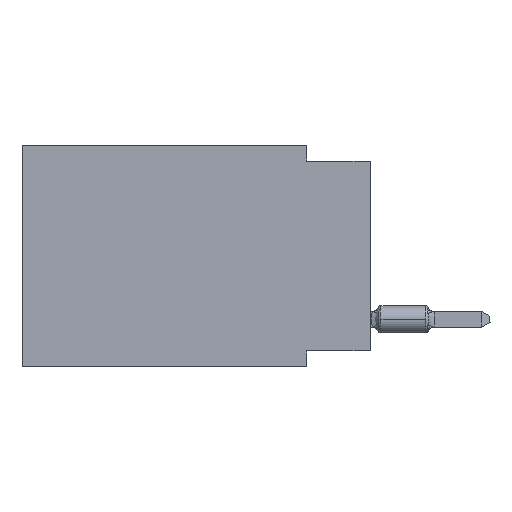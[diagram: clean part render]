
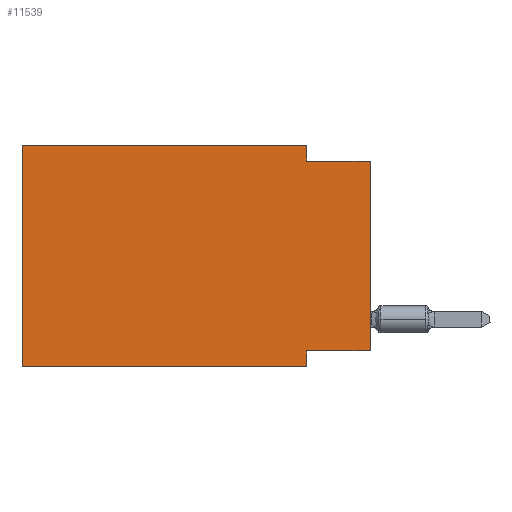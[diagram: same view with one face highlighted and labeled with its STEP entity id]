
A CAD part, left-side view. The second image highlights one B-rep face of the part: STEP entity #11539.
In plain terms, the highlighted planar face has unit normal (-1, 0, 0).
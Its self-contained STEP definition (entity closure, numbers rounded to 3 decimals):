
#651 = DIRECTION ( 'NONE',  ( 0., -1., 0. ) ) ;
#812 = VECTOR ( 'NONE', #651, 1000. ) ;
#1821 = DIRECTION ( 'NONE',  ( 0., -1., 0. ) ) ;
#2051 = LINE ( 'NONE', #42068, #29539 ) ;
#3087 = ORIENTED_EDGE ( 'NONE', *, *, #17412, .F. ) ;
#3097 = AXIS2_PLACEMENT_3D ( 'NONE', #10239, #26311, #42334 ) ;
#3133 = DIRECTION ( 'NONE',  ( 0., 1., 0. ) ) ;
#3184 = DIRECTION ( 'NONE',  ( 0., 0., -1. ) ) ;
#4535 = CARTESIAN_POINT ( 'NONE',  ( 0., 13.97, 0. ) ) ;
#7251 = VECTOR ( 'NONE', #44217, 1000. ) ;
#7357 = LINE ( 'NONE', #51108, #7251 ) ;
#8420 = EDGE_LOOP ( 'NONE', ( #13441, #24797, #3087, #15467, #47632, #21876, #37852, #10080 ) ) ;
#9853 = VERTEX_POINT ( 'NONE', #50223 ) ;
#9971 = FACE_OUTER_BOUND ( 'NONE', #8420, .T. ) ;
#10080 = ORIENTED_EDGE ( 'NONE', *, *, #19672, .F. ) ;
#10239 = CARTESIAN_POINT ( 'NONE',  ( 0., 13.97, 0. ) ) ;
#11117 = CARTESIAN_POINT ( 'NONE',  ( 0., 2.54, -8.89 ) ) ;
#11539 = ADVANCED_FACE ( 'NONE', ( #9971 ), #50274, .F. ) ;
#12179 = LINE ( 'NONE', #4535, #29441 ) ;
#13441 = ORIENTED_EDGE ( 'NONE', *, *, #16770, .T. ) ;
#15467 = ORIENTED_EDGE ( 'NONE', *, *, #21159, .F. ) ;
#16770 = EDGE_CURVE ( 'NONE', #9853, #38584, #48499, .T. ) ;
#17412 = EDGE_CURVE ( 'NONE', #38426, #38122, #2051, .T. ) ;
#19394 = VECTOR ( 'NONE', #1821, 1000. ) ;
#19672 = EDGE_CURVE ( 'NONE', #9853, #25596, #27143, .T. ) ;
#20947 = CARTESIAN_POINT ( 'NONE',  ( 0., 13.97, -8.89 ) ) ;
#21159 = EDGE_CURVE ( 'NONE', #42649, #38426, #7357, .T. ) ;
#21876 = ORIENTED_EDGE ( 'NONE', *, *, #35443, .T. ) ;
#23756 = DIRECTION ( 'NONE',  ( 0., 0., 1. ) ) ;
#24535 = CARTESIAN_POINT ( 'NONE',  ( 0., 2.54, -8.89 ) ) ;
#24567 = DIRECTION ( 'NONE',  ( 0., 0., 1. ) ) ;
#24797 = ORIENTED_EDGE ( 'NONE', *, *, #30691, .F. ) ;
#25596 = VERTEX_POINT ( 'NONE', #35526 ) ;
#26311 = DIRECTION ( 'NONE',  ( 1., 0., 0. ) ) ;
#26814 = DIRECTION ( 'NONE',  ( 0., 0., -1. ) ) ;
#26870 = CARTESIAN_POINT ( 'NONE',  ( 0., 0., -8.255 ) ) ;
#27143 = LINE ( 'NONE', #26870, #38377 ) ;
#27979 = CARTESIAN_POINT ( 'NONE',  ( 0., 0., 0. ) ) ;
#29202 = VECTOR ( 'NONE', #3184, 1000. ) ;
#29441 = VECTOR ( 'NONE', #24567, 1000. ) ;
#29539 = VECTOR ( 'NONE', #26814, 1000. ) ;
#30691 = EDGE_CURVE ( 'NONE', #38122, #38584, #36422, .T. ) ;
#33011 = VERTEX_POINT ( 'NONE', #33751 ) ;
#33751 = CARTESIAN_POINT ( 'NONE',  ( 0., 13.97, -8.89 ) ) ;
#34178 = CARTESIAN_POINT ( 'NONE',  ( 0., 0., -0.635 ) ) ;
#35443 = EDGE_CURVE ( 'NONE', #33011, #41520, #41466, .T. ) ;
#35526 = CARTESIAN_POINT ( 'NONE',  ( 0., 2.54, -8.255 ) ) ;
#36422 = LINE ( 'NONE', #45552, #19394 ) ;
#37476 = CARTESIAN_POINT ( 'NONE',  ( 0., 2.54, -0.635 ) ) ;
#37852 = ORIENTED_EDGE ( 'NONE', *, *, #41389, .F. ) ;
#38122 = VERTEX_POINT ( 'NONE', #37476 ) ;
#38377 = VECTOR ( 'NONE', #3133, 1000. ) ;
#38426 = VERTEX_POINT ( 'NONE', #48263 ) ;
#38503 = EDGE_CURVE ( 'NONE', #33011, #42649, #12179, .T. ) ;
#38584 = VERTEX_POINT ( 'NONE', #34178 ) ;
#41062 = CARTESIAN_POINT ( 'NONE',  ( 0., 13.97, 0. ) ) ;
#41389 = EDGE_CURVE ( 'NONE', #25596, #41520, #51157, .T. ) ;
#41466 = LINE ( 'NONE', #20947, #812 ) ;
#41520 = VERTEX_POINT ( 'NONE', #24535 ) ;
#42068 = CARTESIAN_POINT ( 'NONE',  ( 0., 2.54, 0. ) ) ;
#42334 = DIRECTION ( 'NONE',  ( 0., 0., -1. ) ) ;
#42649 = VERTEX_POINT ( 'NONE', #41062 ) ;
#44217 = DIRECTION ( 'NONE',  ( 0., -1., 0. ) ) ;
#45552 = CARTESIAN_POINT ( 'NONE',  ( 0., 0., -0.635 ) ) ;
#47632 = ORIENTED_EDGE ( 'NONE', *, *, #38503, .F. ) ;
#48263 = CARTESIAN_POINT ( 'NONE',  ( 0., 2.54, 0. ) ) ;
#48499 = LINE ( 'NONE', #27979, #48940 ) ;
#48940 = VECTOR ( 'NONE', #23756, 1000. ) ;
#50223 = CARTESIAN_POINT ( 'NONE',  ( 0., 0., -8.255 ) ) ;
#50274 = PLANE ( 'NONE',  #3097 ) ;
#51108 = CARTESIAN_POINT ( 'NONE',  ( 0., 13.97, 0. ) ) ;
#51157 = LINE ( 'NONE', #11117, #29202 ) ;
